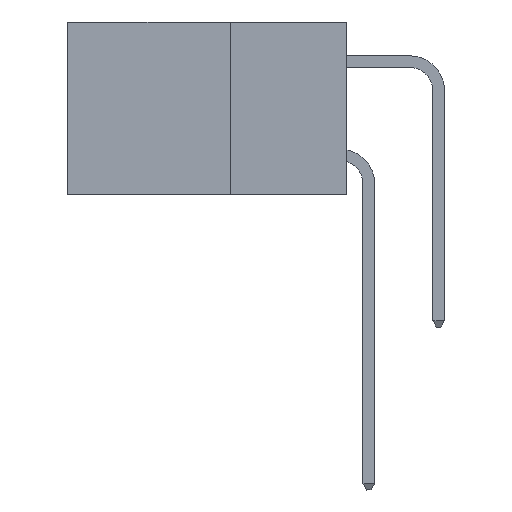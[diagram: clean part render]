
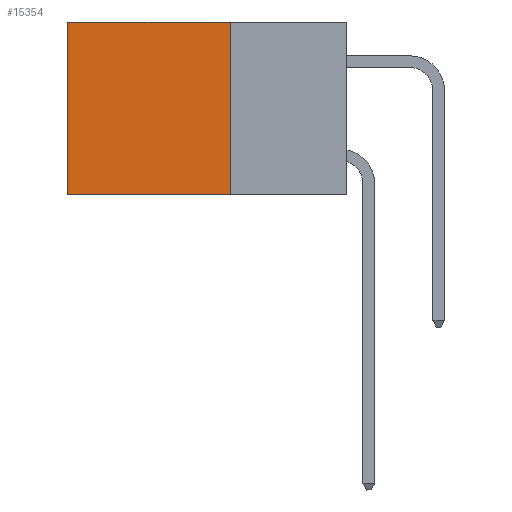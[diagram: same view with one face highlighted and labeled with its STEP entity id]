
A CAD part, left-side view. The second image highlights one B-rep face of the part: STEP entity #15354.
In plain terms, the highlighted planar face has unit normal (-1, 0, 0).
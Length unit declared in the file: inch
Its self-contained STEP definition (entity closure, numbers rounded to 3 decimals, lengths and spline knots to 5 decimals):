
#509 = CARTESIAN_POINT ( 'NONE',  ( 0.2875, 0.25, 0. ) ) ;
#1311 = CARTESIAN_POINT ( 'NONE',  ( 0.2875, 0.25, 0. ) ) ;
#1696 = EDGE_LOOP ( 'NONE', ( #9355, #11459, #12469, #14025 ) ) ;
#2107 = VERTEX_POINT ( 'NONE', #10443 ) ;
#2338 = VECTOR ( 'NONE', #4067, 39.37008 ) ;
#2735 = DIRECTION ( 'NONE',  ( 0., 0., -1. ) ) ;
#3625 = DIRECTION ( 'NONE',  ( 0., 1., 0. ) ) ;
#3835 = EDGE_CURVE ( 'NONE', #2107, #17590, #9900, .T. ) ;
#4067 = DIRECTION ( 'NONE',  ( 0., 0., -1. ) ) ;
#4268 = CARTESIAN_POINT ( 'NONE',  ( 0.2875, 0.25, 0. ) ) ;
#5104 = VERTEX_POINT ( 'NONE', #4268 ) ;
#6104 = EDGE_CURVE ( 'NONE', #5104, #2107, #14841, .T. ) ;
#6232 = CARTESIAN_POINT ( 'NONE',  ( 0.2875, 0.25, -0.37 ) ) ;
#6600 = VECTOR ( 'NONE', #9009, 39.37008 ) ;
#6768 = LINE ( 'NONE', #12168, #13806 ) ;
#8289 = CARTESIAN_POINT ( 'NONE',  ( 0.2875, 0.6, 0. ) ) ;
#9009 = DIRECTION ( 'NONE',  ( 0., 0., -1. ) ) ;
#9214 = CARTESIAN_POINT ( 'NONE',  ( 0.2875, 0.25, 0. ) ) ;
#9355 = ORIENTED_EDGE ( 'NONE', *, *, #3835, .T. ) ;
#9900 = LINE ( 'NONE', #8289, #2338 ) ;
#10378 = LINE ( 'NONE', #509, #6600 ) ;
#10443 = CARTESIAN_POINT ( 'NONE',  ( 0.2875, 0.6, 0. ) ) ;
#10637 = DIRECTION ( 'NONE',  ( 0., 1., 0. ) ) ;
#11217 = DIRECTION ( 'NONE',  ( 1., 0., 0. ) ) ;
#11459 = ORIENTED_EDGE ( 'NONE', *, *, #18218, .F. ) ;
#11610 = EDGE_CURVE ( 'NONE', #5104, #13664, #10378, .T. ) ;
#11760 = FACE_OUTER_BOUND ( 'NONE', #1696, .T. ) ;
#12168 = CARTESIAN_POINT ( 'NONE',  ( 0.2875, 0.25, -0.37 ) ) ;
#12469 = ORIENTED_EDGE ( 'NONE', *, *, #11610, .F. ) ;
#13664 = VERTEX_POINT ( 'NONE', #6232 ) ;
#13806 = VECTOR ( 'NONE', #3625, 39.37008 ) ;
#14025 = ORIENTED_EDGE ( 'NONE', *, *, #6104, .T. ) ;
#14841 = LINE ( 'NONE', #9214, #18125 ) ;
#15354 = ADVANCED_FACE ( 'NONE', ( #11760 ), #18269, .F. ) ;
#16122 = CARTESIAN_POINT ( 'NONE',  ( 0.2875, 0.6, -0.37 ) ) ;
#16709 = AXIS2_PLACEMENT_3D ( 'NONE', #1311, #11217, #2735 ) ;
#17590 = VERTEX_POINT ( 'NONE', #16122 ) ;
#18125 = VECTOR ( 'NONE', #10637, 39.37008 ) ;
#18218 = EDGE_CURVE ( 'NONE', #13664, #17590, #6768, .T. ) ;
#18269 = PLANE ( 'NONE',  #16709 ) ;
